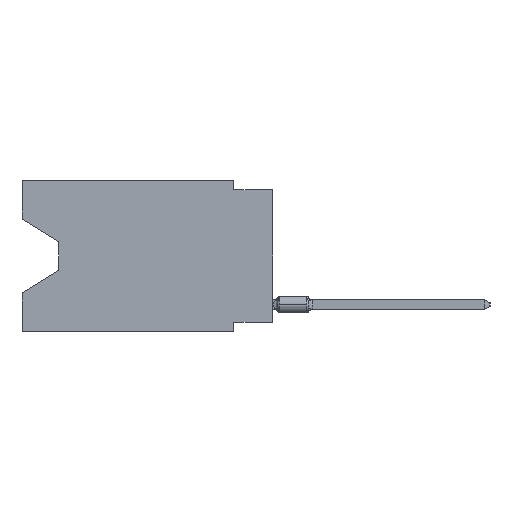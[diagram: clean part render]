
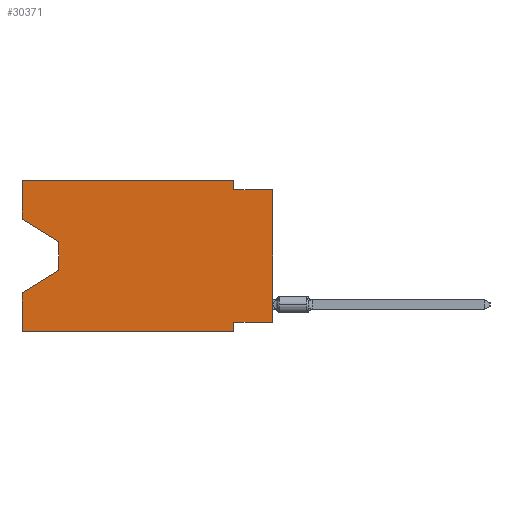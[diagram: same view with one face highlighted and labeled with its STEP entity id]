
A CAD part, left-side view. The second image highlights one B-rep face of the part: STEP entity #30371.
In plain terms, the highlighted planar face has unit normal (-1, 0, 0).
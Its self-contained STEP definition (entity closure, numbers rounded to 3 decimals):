
#279 = CARTESIAN_POINT ( 'NONE',  ( 0., 16.383, -9.906 ) ) ;
#354 = VECTOR ( 'NONE', #386, 1000. ) ;
#386 = DIRECTION ( 'NONE',  ( 0., 0., -1. ) ) ;
#686 = DIRECTION ( 'NONE',  ( 0., 0., -1. ) ) ;
#839 = CARTESIAN_POINT ( 'NONE',  ( 0., 2.54, -0.635 ) ) ;
#1080 = ORIENTED_EDGE ( 'NONE', *, *, #4865, .F. ) ;
#1110 = DIRECTION ( 'NONE',  ( 1., 0., 0. ) ) ;
#1188 = VERTEX_POINT ( 'NONE', #14323 ) ;
#1293 = VERTEX_POINT ( 'NONE', #13790 ) ;
#1484 = CARTESIAN_POINT ( 'NONE',  ( 0., 0., -0.635 ) ) ;
#1999 = CARTESIAN_POINT ( 'NONE',  ( 0., 0., 0. ) ) ;
#2022 = VECTOR ( 'NONE', #31319, 1000. ) ;
#2523 = EDGE_CURVE ( 'NONE', #3420, #23077, #27905, .T. ) ;
#2556 = CARTESIAN_POINT ( 'NONE',  ( 0., 16.383, 0. ) ) ;
#2748 = EDGE_CURVE ( 'NONE', #30233, #1188, #15743, .T. ) ;
#2865 = VERTEX_POINT ( 'NONE', #14502 ) ;
#3294 = VECTOR ( 'NONE', #12530, 1000. ) ;
#3420 = VERTEX_POINT ( 'NONE', #25349 ) ;
#3495 = EDGE_CURVE ( 'NONE', #1293, #34479, #32238, .T. ) ;
#3511 = ORIENTED_EDGE ( 'NONE', *, *, #23758, .T. ) ;
#3759 = PLANE ( 'NONE',  #5719 ) ;
#4643 = LINE ( 'NONE', #10076, #21391 ) ;
#4865 = EDGE_CURVE ( 'NONE', #30233, #23406, #20251, .T. ) ;
#4968 = VERTEX_POINT ( 'NONE', #1484 ) ;
#5140 = VECTOR ( 'NONE', #22462, 1000. ) ;
#5161 = DIRECTION ( 'NONE',  ( 0., 0., 1. ) ) ;
#5226 = CARTESIAN_POINT ( 'NONE',  ( 0., 16.383, -2.546 ) ) ;
#5719 = AXIS2_PLACEMENT_3D ( 'NONE', #25172, #1110, #11801 ) ;
#7185 = CARTESIAN_POINT ( 'NONE',  ( 0., 16.383, 0. ) ) ;
#7464 = VECTOR ( 'NONE', #32407, 1000. ) ;
#9713 = ORIENTED_EDGE ( 'NONE', *, *, #30121, .F. ) ;
#10076 = CARTESIAN_POINT ( 'NONE',  ( 0., 16.383, 0. ) ) ;
#11621 = LINE ( 'NONE', #11787, #354 ) ;
#11736 = CARTESIAN_POINT ( 'NONE',  ( 0., 2.54, 0. ) ) ;
#11787 = CARTESIAN_POINT ( 'NONE',  ( 0., 2.54, -9.906 ) ) ;
#11801 = DIRECTION ( 'NONE',  ( 0., 0., -1. ) ) ;
#12530 = DIRECTION ( 'NONE',  ( 0., 0., 1. ) ) ;
#12666 = VERTEX_POINT ( 'NONE', #24762 ) ;
#12697 = LINE ( 'NONE', #20594, #2022 ) ;
#12975 = CARTESIAN_POINT ( 'NONE',  ( 0., 13.97, -5.893 ) ) ;
#13754 = ORIENTED_EDGE ( 'NONE', *, *, #3495, .T. ) ;
#13790 = CARTESIAN_POINT ( 'NONE',  ( 0., 16.383, -9.906 ) ) ;
#14323 = CARTESIAN_POINT ( 'NONE',  ( 0., 13.97, -4.013 ) ) ;
#14347 = EDGE_CURVE ( 'NONE', #23077, #4968, #12697, .T. ) ;
#14502 = CARTESIAN_POINT ( 'NONE',  ( 0., 2.54, -9.271 ) ) ;
#14601 = EDGE_CURVE ( 'NONE', #2865, #34479, #11621, .T. ) ;
#15511 = LINE ( 'NONE', #1999, #3294 ) ;
#15743 = LINE ( 'NONE', #5226, #33791 ) ;
#17534 = CARTESIAN_POINT ( 'NONE',  ( 0., 13.97, -5.893 ) ) ;
#19114 = LINE ( 'NONE', #32645, #5140 ) ;
#19465 = ORIENTED_EDGE ( 'NONE', *, *, #21346, .T. ) ;
#20251 = LINE ( 'NONE', #23899, #28304 ) ;
#20349 = ORIENTED_EDGE ( 'NONE', *, *, #32260, .F. ) ;
#20594 = CARTESIAN_POINT ( 'NONE',  ( 0., 0., -0.635 ) ) ;
#21346 = EDGE_CURVE ( 'NONE', #26247, #22913, #26850, .T. ) ;
#21391 = VECTOR ( 'NONE', #5161, 1000. ) ;
#22031 = DIRECTION ( 'NONE',  ( 0., 0., -1. ) ) ;
#22305 = VECTOR ( 'NONE', #25971, 1000. ) ;
#22462 = DIRECTION ( 'NONE',  ( 0., 1., 0. ) ) ;
#22551 = VECTOR ( 'NONE', #686, 1000. ) ;
#22683 = ORIENTED_EDGE ( 'NONE', *, *, #14347, .F. ) ;
#22771 = EDGE_CURVE ( 'NONE', #12666, #2865, #19114, .T. ) ;
#22913 = VERTEX_POINT ( 'NONE', #30552 ) ;
#23077 = VERTEX_POINT ( 'NONE', #839 ) ;
#23406 = VERTEX_POINT ( 'NONE', #2556 ) ;
#23639 = EDGE_LOOP ( 'NONE', ( #34233, #24968, #19465, #9713, #13754, #34493, #32981, #3511, #22683, #28907, #20349, #1080 ) ) ;
#23758 = EDGE_CURVE ( 'NONE', #12666, #4968, #15511, .T. ) ;
#23899 = CARTESIAN_POINT ( 'NONE',  ( 0., 16.383, 0. ) ) ;
#24527 = DIRECTION ( 'NONE',  ( 0., -0.855, -0.519 ) ) ;
#24762 = CARTESIAN_POINT ( 'NONE',  ( 0., 0., -9.271 ) ) ;
#24968 = ORIENTED_EDGE ( 'NONE', *, *, #33033, .T. ) ;
#25172 = CARTESIAN_POINT ( 'NONE',  ( 0., 16.383, 0. ) ) ;
#25349 = CARTESIAN_POINT ( 'NONE',  ( 0., 2.54, 0. ) ) ;
#25795 = LINE ( 'NONE', #7185, #22305 ) ;
#25971 = DIRECTION ( 'NONE',  ( 0., -1., 0. ) ) ;
#25983 = VECTOR ( 'NONE', #22031, 1000. ) ;
#26247 = VERTEX_POINT ( 'NONE', #17534 ) ;
#26850 = LINE ( 'NONE', #12975, #31621 ) ;
#26945 = CARTESIAN_POINT ( 'NONE',  ( 0., 13.97, -4.013 ) ) ;
#27810 = FACE_OUTER_BOUND ( 'NONE', #23639, .T. ) ;
#27905 = LINE ( 'NONE', #11736, #22551 ) ;
#28170 = CARTESIAN_POINT ( 'NONE',  ( 0., 2.54, -9.906 ) ) ;
#28304 = VECTOR ( 'NONE', #34595, 1000. ) ;
#28907 = ORIENTED_EDGE ( 'NONE', *, *, #2523, .F. ) ;
#30121 = EDGE_CURVE ( 'NONE', #1293, #22913, #4643, .T. ) ;
#30233 = VERTEX_POINT ( 'NONE', #32190 ) ;
#30371 = ADVANCED_FACE ( 'NONE', ( #27810 ), #3759, .F. ) ;
#30552 = CARTESIAN_POINT ( 'NONE',  ( 0., 16.383, -7.36 ) ) ;
#31319 = DIRECTION ( 'NONE',  ( 0., -1., 0. ) ) ;
#31621 = VECTOR ( 'NONE', #31941, 1000. ) ;
#31941 = DIRECTION ( 'NONE',  ( 0., 0.855, -0.519 ) ) ;
#32190 = CARTESIAN_POINT ( 'NONE',  ( 0., 16.383, -2.546 ) ) ;
#32219 = LINE ( 'NONE', #26945, #25983 ) ;
#32238 = LINE ( 'NONE', #279, #7464 ) ;
#32260 = EDGE_CURVE ( 'NONE', #23406, #3420, #25795, .T. ) ;
#32407 = DIRECTION ( 'NONE',  ( 0., -1., 0. ) ) ;
#32645 = CARTESIAN_POINT ( 'NONE',  ( 0., 0., -9.271 ) ) ;
#32981 = ORIENTED_EDGE ( 'NONE', *, *, #22771, .F. ) ;
#33033 = EDGE_CURVE ( 'NONE', #1188, #26247, #32219, .T. ) ;
#33791 = VECTOR ( 'NONE', #24527, 1000. ) ;
#34233 = ORIENTED_EDGE ( 'NONE', *, *, #2748, .T. ) ;
#34479 = VERTEX_POINT ( 'NONE', #28170 ) ;
#34493 = ORIENTED_EDGE ( 'NONE', *, *, #14601, .F. ) ;
#34595 = DIRECTION ( 'NONE',  ( 0., 0., 1. ) ) ;
